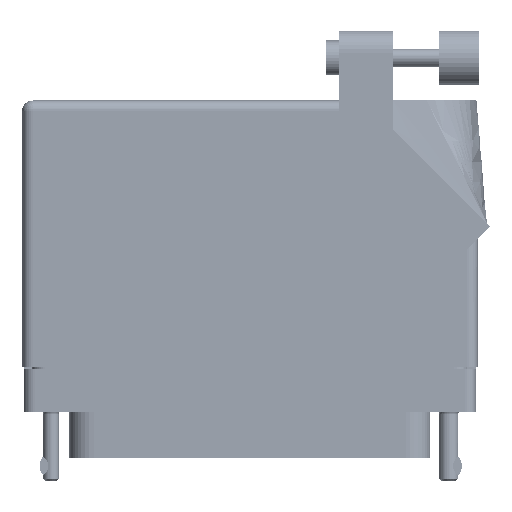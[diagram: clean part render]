
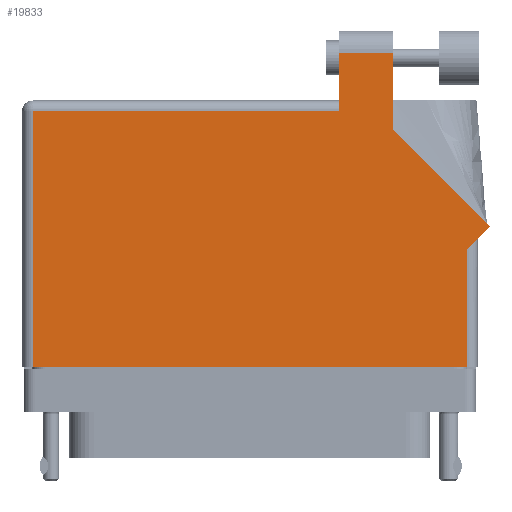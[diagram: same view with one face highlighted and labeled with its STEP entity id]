
A CAD part, front view. The second image highlights one B-rep face of the part: STEP entity #19833.
In plain terms, the highlighted face is planar.
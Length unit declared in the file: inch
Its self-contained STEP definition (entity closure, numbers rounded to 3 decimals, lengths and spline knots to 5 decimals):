
#658 = ORIENTED_EDGE ( 'NONE', *, *, #3755, .T. ) ;
#3755 = EDGE_CURVE ( 'NONE', #16646, #37420, #41822, .T. ) ;
#3779 = CARTESIAN_POINT ( 'NONE',  ( 0.513, 1.705, 0.455 ) ) ;
#4348 = DIRECTION ( 'NONE',  ( 0., 1., 0. ) ) ;
#4778 = LINE ( 'NONE', #35726, #45378 ) ;
#5005 = VECTOR ( 'NONE', #55126, 39.37008 ) ;
#5127 = VECTOR ( 'NONE', #14265, 39.37008 ) ;
#6848 = EDGE_CURVE ( 'NONE', #42498, #39209, #17150, .T. ) ;
#7385 = EDGE_CURVE ( 'NONE', #34780, #16646, #45938, .T. ) ;
#7586 = CARTESIAN_POINT ( 'NONE',  ( -1.306, 1.43, 0.455 ) ) ;
#7668 = ORIENTED_EDGE ( 'NONE', *, *, #35602, .T. ) ;
#8871 = VECTOR ( 'NONE', #4348, 39.37008 ) ;
#9084 = CARTESIAN_POINT ( 'NONE',  ( -1.244, -0.1, 0.455 ) ) ;
#9572 = DIRECTION ( 'NONE',  ( 0., -1., 0. ) ) ;
#13435 = CARTESIAN_POINT ( 'NONE',  ( -1.306, -0.1, 0.455 ) ) ;
#13739 = CARTESIAN_POINT ( 'NONE',  ( 0.513, 1.705, 0.455 ) ) ;
#14265 = DIRECTION ( 'NONE',  ( 0., 1., 0. ) ) ;
#14508 = CARTESIAN_POINT ( 'NONE',  ( 0.513, 1.43, 0.455 ) ) ;
#16381 = ORIENTED_EDGE ( 'NONE', *, *, #49349, .T. ) ;
#16646 = VERTEX_POINT ( 'NONE', #9084 ) ;
#17150 = LINE ( 'NONE', #39959, #26765 ) ;
#18399 = CARTESIAN_POINT ( 'NONE',  ( 1.244, 0.575, 0.455 ) ) ;
#19833 = ADVANCED_FACE ( 'NONE', ( #52377 ), #22243, .F. ) ;
#20718 = ORIENTED_EDGE ( 'NONE', *, *, #6848, .T. ) ;
#21488 = LINE ( 'NONE', #42717, #8871 ) ;
#21646 = LINE ( 'NONE', #14508, #60043 ) ;
#21982 = LINE ( 'NONE', #26997, #5005 ) ;
#22243 = PLANE ( 'NONE',  #54377 ) ;
#23776 = VERTEX_POINT ( 'NONE', #55209 ) ;
#25052 = CARTESIAN_POINT ( 'NONE',  ( -1.244, -0.1, 0.455 ) ) ;
#25288 = EDGE_LOOP ( 'NONE', ( #56409, #33232, #57687, #51539, #59078, #658, #16381, #20718, #7668 ) ) ;
#25757 = LINE ( 'NONE', #51912, #5127 ) ;
#26241 = CARTESIAN_POINT ( 'NONE',  ( 1.37671, 0.70771, 0.455 ) ) ;
#26765 = VECTOR ( 'NONE', #35818, 39.37008 ) ;
#26997 = CARTESIAN_POINT ( 'NONE',  ( 1.37671, 0.70771, 0.455 ) ) ;
#28557 = CARTESIAN_POINT ( 'NONE',  ( -1.244, 1.368, 0.455 ) ) ;
#30786 = CARTESIAN_POINT ( 'NONE',  ( 0.513, 1.368, 0.455 ) ) ;
#31547 = VERTEX_POINT ( 'NONE', #30786 ) ;
#32165 = EDGE_CURVE ( 'NONE', #46481, #31547, #21646, .T. ) ;
#33232 = ORIENTED_EDGE ( 'NONE', *, *, #36199, .T. ) ;
#34780 = VERTEX_POINT ( 'NONE', #28557 ) ;
#35250 = VECTOR ( 'NONE', #51586, 39.37008 ) ;
#35602 = EDGE_CURVE ( 'NONE', #39209, #36273, #21982, .T. ) ;
#35726 = CARTESIAN_POINT ( 'NONE',  ( -1.306, 1.368, 0.455 ) ) ;
#35818 = DIRECTION ( 'NONE',  ( 0.707, 0.707, 0. ) ) ;
#36199 = EDGE_CURVE ( 'NONE', #23776, #46481, #60425, .T. ) ;
#36273 = VERTEX_POINT ( 'NONE', #46960 ) ;
#37420 = VERTEX_POINT ( 'NONE', #52339 ) ;
#39209 = VERTEX_POINT ( 'NONE', #26241 ) ;
#39221 = EDGE_CURVE ( 'NONE', #31547, #34780, #4778, .T. ) ;
#39959 = CARTESIAN_POINT ( 'NONE',  ( 1.306, 0.637, 0.455 ) ) ;
#40809 = DIRECTION ( 'NONE',  ( 0., 0., -1. ) ) ;
#41822 = LINE ( 'NONE', #13435, #46293 ) ;
#42498 = VERTEX_POINT ( 'NONE', #18399 ) ;
#42575 = EDGE_CURVE ( 'NONE', #36273, #23776, #25757, .T. ) ;
#42717 = CARTESIAN_POINT ( 'NONE',  ( 1.244, 0.637, 0.455 ) ) ;
#45378 = VECTOR ( 'NONE', #59916, 39.37008 ) ;
#45938 = LINE ( 'NONE', #25052, #57070 ) ;
#46293 = VECTOR ( 'NONE', #59967, 39.37008 ) ;
#46481 = VERTEX_POINT ( 'NONE', #3779 ) ;
#46960 = CARTESIAN_POINT ( 'NONE',  ( 0.82, 1.26442, 0.455 ) ) ;
#49349 = EDGE_CURVE ( 'NONE', #37420, #42498, #21488, .T. ) ;
#51539 = ORIENTED_EDGE ( 'NONE', *, *, #39221, .T. ) ;
#51586 = DIRECTION ( 'NONE',  ( -1., 0., 0. ) ) ;
#51912 = CARTESIAN_POINT ( 'NONE',  ( 0.82, 1.26442, 0.455 ) ) ;
#52339 = CARTESIAN_POINT ( 'NONE',  ( 1.244, -0.1, 0.455 ) ) ;
#52377 = FACE_OUTER_BOUND ( 'NONE', #25288, .T. ) ;
#54377 = AXIS2_PLACEMENT_3D ( 'NONE', #7586, #40809, #54899 ) ;
#54899 = DIRECTION ( 'NONE',  ( -1., 0., 0. ) ) ;
#55126 = DIRECTION ( 'NONE',  ( -0.707, 0.707, 0. ) ) ;
#55209 = CARTESIAN_POINT ( 'NONE',  ( 0.82, 1.705, 0.455 ) ) ;
#56409 = ORIENTED_EDGE ( 'NONE', *, *, #42575, .T. ) ;
#57070 = VECTOR ( 'NONE', #58334, 39.37008 ) ;
#57687 = ORIENTED_EDGE ( 'NONE', *, *, #32165, .T. ) ;
#58334 = DIRECTION ( 'NONE',  ( 0., -1., 0. ) ) ;
#59078 = ORIENTED_EDGE ( 'NONE', *, *, #7385, .T. ) ;
#59916 = DIRECTION ( 'NONE',  ( -1., 0., 0. ) ) ;
#59967 = DIRECTION ( 'NONE',  ( 1., 0., 0. ) ) ;
#60043 = VECTOR ( 'NONE', #9572, 39.37008 ) ;
#60425 = LINE ( 'NONE', #13739, #35250 ) ;
